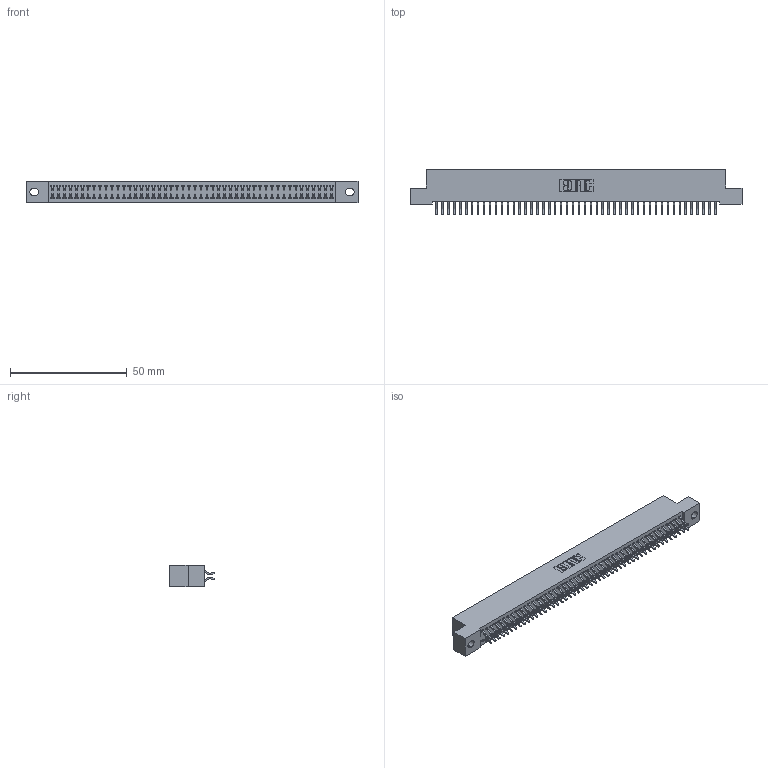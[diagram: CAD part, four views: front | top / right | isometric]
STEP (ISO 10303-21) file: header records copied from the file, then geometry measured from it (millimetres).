
FILE_DESCRIPTION (( 'STEP AP203' ), '1' );
FILE_NAME ('342-096-556-202.STEP', '2019-10-04T16:16:21', ( '' ), ( '' ), 'SwSTEP 2.0', 'SolidWorks 2016', '' );
FILE_SCHEMA (( 'CONFIG_CONTROL_DESIGN' ));
Length unit declared in the file: inch
Products named in the file (3): 342-096-556-202; 342 Part_.128 Slot; 345-292-001_556 Tail
Assembly tree (97 placements, depth 2):
  342-096-556-202
    342 Part_.128 Slot
    345-292-001_556 Tail  x96
Bounding box: 142.24 x 19.58 x 9.4 mm (x, y, z)
Volume: 12754.1 mm3; surface area: 20574.6 mm2
Topology: 97 solids, 97 shells, 5682 faces, 16919 edges, 11150 vertices
Faces by surface type: plane 3910, cylinder 1772
Entity records: 30327 total; most frequent: CARTESIAN_POINT 5034, ORIENTED_EDGE 4958, DIRECTION 4279, EDGE_CURVE 2479, LINE 2343, VECTOR 2343, VERTEX_POINT 1650, AXIS2_PLACEMENT_3D 968
